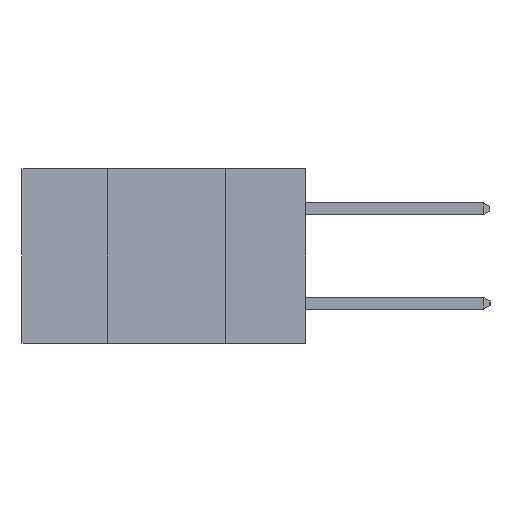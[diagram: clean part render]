
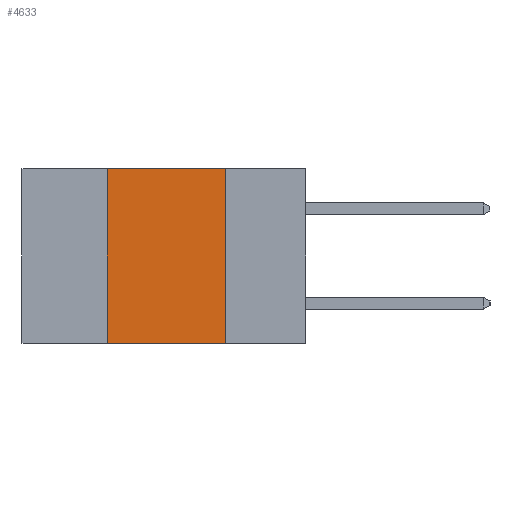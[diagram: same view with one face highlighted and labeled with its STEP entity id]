
A CAD part, left-side view. The second image highlights one B-rep face of the part: STEP entity #4633.
In plain terms, the highlighted planar face has unit normal (-1, 0, 0).
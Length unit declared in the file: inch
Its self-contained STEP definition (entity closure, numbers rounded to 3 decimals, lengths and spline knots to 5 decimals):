
#123 = LINE ( 'NONE', #1317, #1708 ) ;
#265 = ORIENTED_EDGE ( 'NONE', *, *, #7310, .F. ) ;
#360 = CARTESIAN_POINT ( 'NONE',  ( 0., 0.17, -0.37 ) ) ;
#849 = DIRECTION ( 'NONE',  ( 0., 0., -1. ) ) ;
#1048 = DIRECTION ( 'NONE',  ( 0., -1., 0. ) ) ;
#1187 = LINE ( 'NONE', #8653, #8796 ) ;
#1317 = CARTESIAN_POINT ( 'NONE',  ( 0., 0.42, -0.37 ) ) ;
#1708 = VECTOR ( 'NONE', #7435, 39.37008 ) ;
#2360 = DIRECTION ( 'NONE',  ( 0., 0., -1. ) ) ;
#2396 = DIRECTION ( 'NONE',  ( 1., 0., 0. ) ) ;
#2420 = CARTESIAN_POINT ( 'NONE',  ( 0., 0.6, 0. ) ) ;
#2564 = VECTOR ( 'NONE', #9078, 39.37008 ) ;
#2641 = PLANE ( 'NONE',  #3285 ) ;
#3001 = VECTOR ( 'NONE', #849, 39.37008 ) ;
#3008 = CARTESIAN_POINT ( 'NONE',  ( 0., 0.6, 0. ) ) ;
#3188 = ORIENTED_EDGE ( 'NONE', *, *, #9277, .F. ) ;
#3263 = ORIENTED_EDGE ( 'NONE', *, *, #9167, .F. ) ;
#3285 = AXIS2_PLACEMENT_3D ( 'NONE', #2420, #2396, #2360 ) ;
#3376 = CARTESIAN_POINT ( 'NONE',  ( 0., 0.42, -0.37 ) ) ;
#4533 = LINE ( 'NONE', #6240, #3001 ) ;
#4633 = ADVANCED_FACE ( 'NONE', ( #6744 ), #2641, .F. ) ;
#5526 = ORIENTED_EDGE ( 'NONE', *, *, #6172, .T. ) ;
#6172 = EDGE_CURVE ( 'NONE', #8940, #7438, #1187, .T. ) ;
#6240 = CARTESIAN_POINT ( 'NONE',  ( 0., 0.17, -0.37 ) ) ;
#6402 = VERTEX_POINT ( 'NONE', #6730 ) ;
#6467 = EDGE_LOOP ( 'NONE', ( #265, #3188, #3263, #5526 ) ) ;
#6598 = VERTEX_POINT ( 'NONE', #9144 ) ;
#6730 = CARTESIAN_POINT ( 'NONE',  ( 0., 0.17, 0. ) ) ;
#6744 = FACE_OUTER_BOUND ( 'NONE', #6467, .T. ) ;
#6910 = LINE ( 'NONE', #3008, #2564 ) ;
#7310 = EDGE_CURVE ( 'NONE', #6402, #7438, #4533, .T. ) ;
#7435 = DIRECTION ( 'NONE',  ( 0., 0., 1. ) ) ;
#7438 = VERTEX_POINT ( 'NONE', #360 ) ;
#8653 = CARTESIAN_POINT ( 'NONE',  ( 0., 0.6, -0.37 ) ) ;
#8796 = VECTOR ( 'NONE', #1048, 39.37008 ) ;
#8940 = VERTEX_POINT ( 'NONE', #3376 ) ;
#9078 = DIRECTION ( 'NONE',  ( 0., -1., 0. ) ) ;
#9144 = CARTESIAN_POINT ( 'NONE',  ( 0., 0.42, 0. ) ) ;
#9167 = EDGE_CURVE ( 'NONE', #8940, #6598, #123, .T. ) ;
#9277 = EDGE_CURVE ( 'NONE', #6598, #6402, #6910, .T. ) ;
